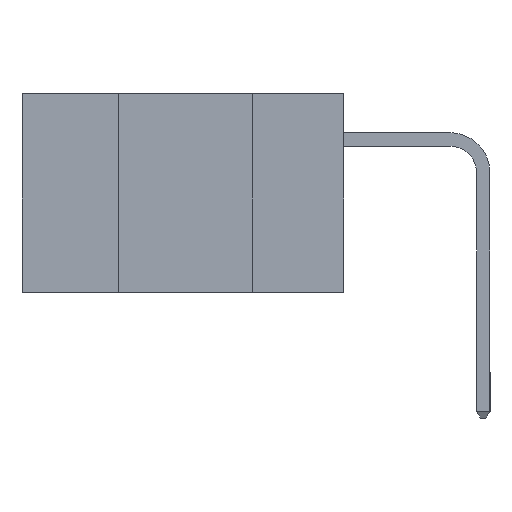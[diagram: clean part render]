
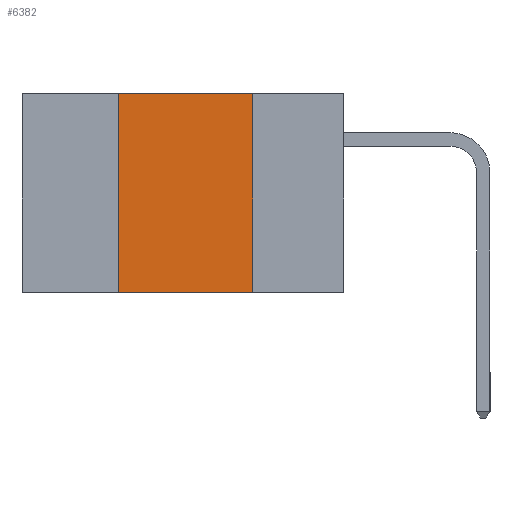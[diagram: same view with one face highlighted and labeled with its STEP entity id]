
A CAD part, left-side view. The second image highlights one B-rep face of the part: STEP entity #6382.
In plain terms, the highlighted planar face has unit normal (-1, 0, 0).
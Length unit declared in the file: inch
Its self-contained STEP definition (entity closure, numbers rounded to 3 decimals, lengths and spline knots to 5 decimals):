
#656 = DIRECTION ( 'NONE',  ( 0., 0., 1. ) ) ;
#891 = VECTOR ( 'NONE', #2422, 39.37008 ) ;
#1303 = CARTESIAN_POINT ( 'NONE',  ( 0., 0.6, -0.37 ) ) ;
#1523 = CARTESIAN_POINT ( 'NONE',  ( 0., 0.17, 0. ) ) ;
#2422 = DIRECTION ( 'NONE',  ( 0., -1., 0. ) ) ;
#3279 = CARTESIAN_POINT ( 'NONE',  ( 0., 0.6, 0. ) ) ;
#3834 = LINE ( 'NONE', #16089, #12411 ) ;
#4018 = LINE ( 'NONE', #6895, #891 ) ;
#4085 = LINE ( 'NONE', #1303, #13234 ) ;
#5292 = ORIENTED_EDGE ( 'NONE', *, *, #6876, .F. ) ;
#5422 = EDGE_CURVE ( 'NONE', #8194, #16438, #4085, .T. ) ;
#6002 = ORIENTED_EDGE ( 'NONE', *, *, #5422, .T. ) ;
#6382 = ADVANCED_FACE ( 'NONE', ( #10930 ), #10839, .F. ) ;
#6876 = EDGE_CURVE ( 'NONE', #12979, #12161, #4018, .T. ) ;
#6895 = CARTESIAN_POINT ( 'NONE',  ( 0., 0.6, 0. ) ) ;
#7853 = DIRECTION ( 'NONE',  ( 0., 0., -1. ) ) ;
#8194 = VERTEX_POINT ( 'NONE', #11604 ) ;
#8514 = EDGE_CURVE ( 'NONE', #8194, #12979, #17251, .T. ) ;
#8926 = CARTESIAN_POINT ( 'NONE',  ( 0., 0.42, 0. ) ) ;
#8940 = CARTESIAN_POINT ( 'NONE',  ( 0., 0.17, -0.37 ) ) ;
#9348 = DIRECTION ( 'NONE',  ( 1., 0., 0. ) ) ;
#10839 = PLANE ( 'NONE',  #14548 ) ;
#10930 = FACE_OUTER_BOUND ( 'NONE', #15149, .T. ) ;
#11441 = EDGE_CURVE ( 'NONE', #12161, #16438, #3834, .T. ) ;
#11604 = CARTESIAN_POINT ( 'NONE',  ( 0., 0.42, -0.37 ) ) ;
#12161 = VERTEX_POINT ( 'NONE', #1523 ) ;
#12411 = VECTOR ( 'NONE', #14380, 39.37008 ) ;
#12860 = CARTESIAN_POINT ( 'NONE',  ( 0., 0.42, -0.37 ) ) ;
#12979 = VERTEX_POINT ( 'NONE', #8926 ) ;
#13234 = VECTOR ( 'NONE', #16338, 39.37008 ) ;
#14380 = DIRECTION ( 'NONE',  ( 0., 0., -1. ) ) ;
#14548 = AXIS2_PLACEMENT_3D ( 'NONE', #3279, #9348, #7853 ) ;
#15149 = EDGE_LOOP ( 'NONE', ( #16099, #5292, #19391, #6002 ) ) ;
#16089 = CARTESIAN_POINT ( 'NONE',  ( 0., 0.17, -0.37 ) ) ;
#16099 = ORIENTED_EDGE ( 'NONE', *, *, #11441, .F. ) ;
#16338 = DIRECTION ( 'NONE',  ( 0., -1., 0. ) ) ;
#16438 = VERTEX_POINT ( 'NONE', #8940 ) ;
#16844 = VECTOR ( 'NONE', #656, 39.37008 ) ;
#17251 = LINE ( 'NONE', #12860, #16844 ) ;
#19391 = ORIENTED_EDGE ( 'NONE', *, *, #8514, .F. ) ;
